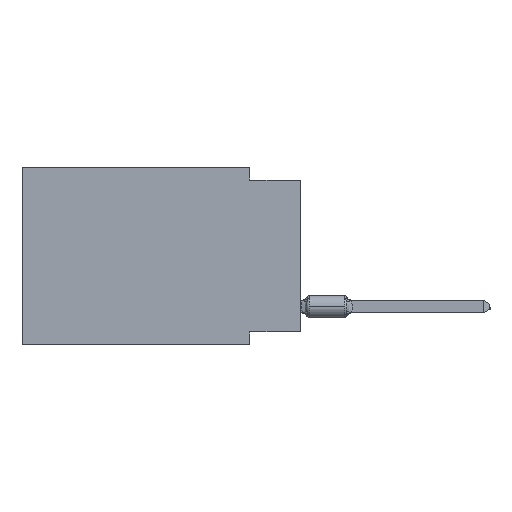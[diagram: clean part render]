
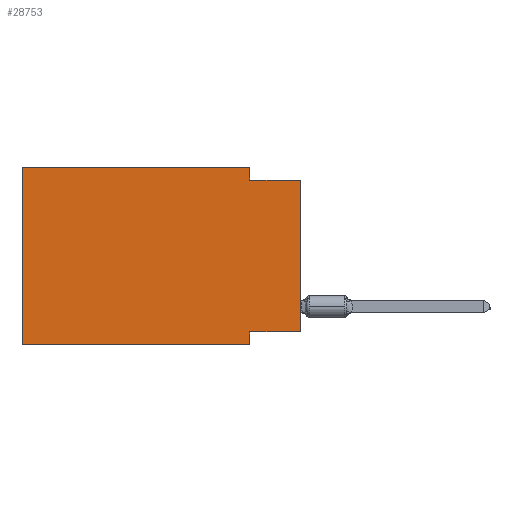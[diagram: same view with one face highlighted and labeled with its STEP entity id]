
A CAD part, left-side view. The second image highlights one B-rep face of the part: STEP entity #28753.
In plain terms, the highlighted planar face has unit normal (-1, 0, 0).
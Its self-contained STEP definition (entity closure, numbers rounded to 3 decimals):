
#135 = VECTOR ( 'NONE', #20785, 1000. ) ;
#816 = DIRECTION ( 'NONE',  ( 0., 0., -1. ) ) ;
#1398 = LINE ( 'NONE', #24962, #17190 ) ;
#1410 = EDGE_LOOP ( 'NONE', ( #27401, #30384, #5000, #6972, #14838, #23605, #11820, #15094 ) ) ;
#1585 = EDGE_CURVE ( 'NONE', #18558, #5497, #14928, .T. ) ;
#3286 = CARTESIAN_POINT ( 'NONE',  ( 0., 2.54, -8.89 ) ) ;
#3396 = CARTESIAN_POINT ( 'NONE',  ( 0., 13.97, -8.89 ) ) ;
#3739 = CARTESIAN_POINT ( 'NONE',  ( 0., 13.97, 0. ) ) ;
#3994 = CARTESIAN_POINT ( 'NONE',  ( 0., 2.54, -0.635 ) ) ;
#4455 = EDGE_CURVE ( 'NONE', #5617, #20261, #21051, .T. ) ;
#4674 = LINE ( 'NONE', #12017, #20643 ) ;
#4936 = EDGE_CURVE ( 'NONE', #30169, #20261, #1398, .T. ) ;
#5000 = ORIENTED_EDGE ( 'NONE', *, *, #16780, .F. ) ;
#5497 = VERTEX_POINT ( 'NONE', #12723 ) ;
#5617 = VERTEX_POINT ( 'NONE', #3994 ) ;
#6513 = CARTESIAN_POINT ( 'NONE',  ( 0., 0., -0.635 ) ) ;
#6972 = ORIENTED_EDGE ( 'NONE', *, *, #10384, .F. ) ;
#7113 = LINE ( 'NONE', #28520, #24791 ) ;
#8340 = PLANE ( 'NONE',  #23782 ) ;
#9427 = CARTESIAN_POINT ( 'NONE',  ( 0., 0., -8.255 ) ) ;
#9961 = CARTESIAN_POINT ( 'NONE',  ( 0., 2.54, 0. ) ) ;
#10001 = VECTOR ( 'NONE', #13851, 1000. ) ;
#10384 = EDGE_CURVE ( 'NONE', #13962, #18106, #7113, .T. ) ;
#10447 = DIRECTION ( 'NONE',  ( 0., -1., 0. ) ) ;
#10618 = VECTOR ( 'NONE', #24524, 1000. ) ;
#10639 = VECTOR ( 'NONE', #10447, 1000. ) ;
#10798 = DIRECTION ( 'NONE',  ( 1., 0., 0. ) ) ;
#11820 = ORIENTED_EDGE ( 'NONE', *, *, #30345, .F. ) ;
#12017 = CARTESIAN_POINT ( 'NONE',  ( 0., 2.54, 0. ) ) ;
#12723 = CARTESIAN_POINT ( 'NONE',  ( 0., 2.54, -8.89 ) ) ;
#13142 = CARTESIAN_POINT ( 'NONE',  ( 0., 2.54, -8.255 ) ) ;
#13851 = DIRECTION ( 'NONE',  ( 0., 0., 1. ) ) ;
#13962 = VERTEX_POINT ( 'NONE', #22979 ) ;
#14838 = ORIENTED_EDGE ( 'NONE', *, *, #28787, .F. ) ;
#14928 = LINE ( 'NONE', #3396, #10639 ) ;
#15094 = ORIENTED_EDGE ( 'NONE', *, *, #25543, .F. ) ;
#16156 = LINE ( 'NONE', #22944, #135 ) ;
#16425 = DIRECTION ( 'NONE',  ( 0., -1., 0. ) ) ;
#16780 = EDGE_CURVE ( 'NONE', #18106, #5617, #4674, .T. ) ;
#16984 = DIRECTION ( 'NONE',  ( 0., 0., 1. ) ) ;
#17190 = VECTOR ( 'NONE', #16984, 1000. ) ;
#18038 = CARTESIAN_POINT ( 'NONE',  ( 0., 13.97, 0. ) ) ;
#18106 = VERTEX_POINT ( 'NONE', #9961 ) ;
#18558 = VERTEX_POINT ( 'NONE', #22680 ) ;
#20202 = DIRECTION ( 'NONE',  ( 0., 0., -1. ) ) ;
#20261 = VERTEX_POINT ( 'NONE', #6513 ) ;
#20643 = VECTOR ( 'NONE', #816, 1000. ) ;
#20785 = DIRECTION ( 'NONE',  ( 0., 1., 0. ) ) ;
#21051 = LINE ( 'NONE', #21506, #21668 ) ;
#21506 = CARTESIAN_POINT ( 'NONE',  ( 0., 0., -0.635 ) ) ;
#21668 = VECTOR ( 'NONE', #16425, 1000. ) ;
#22050 = DIRECTION ( 'NONE',  ( 0., -1., 0. ) ) ;
#22680 = CARTESIAN_POINT ( 'NONE',  ( 0., 13.97, -8.89 ) ) ;
#22821 = FACE_OUTER_BOUND ( 'NONE', #1410, .T. ) ;
#22944 = CARTESIAN_POINT ( 'NONE',  ( 0., 0., -8.255 ) ) ;
#22979 = CARTESIAN_POINT ( 'NONE',  ( 0., 13.97, 0. ) ) ;
#23605 = ORIENTED_EDGE ( 'NONE', *, *, #1585, .T. ) ;
#23782 = AXIS2_PLACEMENT_3D ( 'NONE', #3739, #10798, #20202 ) ;
#24524 = DIRECTION ( 'NONE',  ( 0., 0., -1. ) ) ;
#24791 = VECTOR ( 'NONE', #22050, 1000. ) ;
#24962 = CARTESIAN_POINT ( 'NONE',  ( 0., 0., 0. ) ) ;
#25543 = EDGE_CURVE ( 'NONE', #30169, #27656, #16156, .T. ) ;
#26681 = LINE ( 'NONE', #3286, #10618 ) ;
#27401 = ORIENTED_EDGE ( 'NONE', *, *, #4936, .T. ) ;
#27656 = VERTEX_POINT ( 'NONE', #13142 ) ;
#28520 = CARTESIAN_POINT ( 'NONE',  ( 0., 13.97, 0. ) ) ;
#28753 = ADVANCED_FACE ( 'NONE', ( #22821 ), #8340, .F. ) ;
#28787 = EDGE_CURVE ( 'NONE', #18558, #13962, #29751, .T. ) ;
#29751 = LINE ( 'NONE', #18038, #10001 ) ;
#30169 = VERTEX_POINT ( 'NONE', #9427 ) ;
#30345 = EDGE_CURVE ( 'NONE', #27656, #5497, #26681, .T. ) ;
#30384 = ORIENTED_EDGE ( 'NONE', *, *, #4455, .F. ) ;
